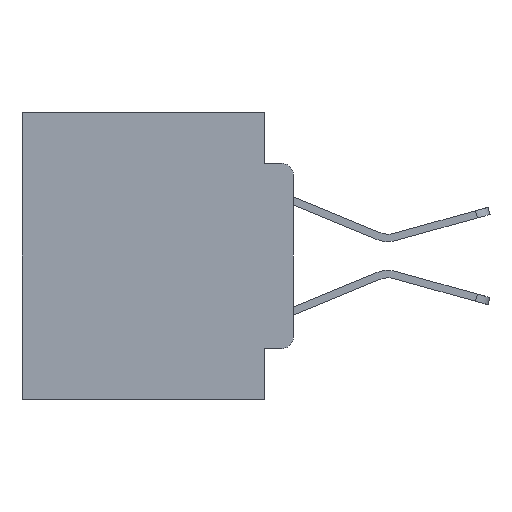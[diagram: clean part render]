
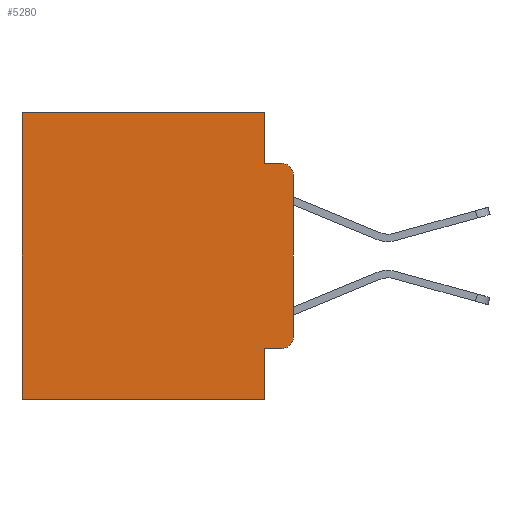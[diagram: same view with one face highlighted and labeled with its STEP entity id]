
A CAD part, left-side view. The second image highlights one B-rep face of the part: STEP entity #5280.
In plain terms, the highlighted planar face has unit normal (-1, 0, 0).
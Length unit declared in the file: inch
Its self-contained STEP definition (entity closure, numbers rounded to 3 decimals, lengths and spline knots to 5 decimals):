
#227 = LINE ( 'NONE', #12690, #11710 ) ;
#474 = LINE ( 'NONE', #9135, #16543 ) ;
#956 = VECTOR ( 'NONE', #20732, 39.37008 ) ;
#1120 = FACE_OUTER_BOUND ( 'NONE', #25612, .T. ) ;
#1221 = VECTOR ( 'NONE', #12861, 39.37008 ) ;
#1805 = VERTEX_POINT ( 'NONE', #17843 ) ;
#2134 = LINE ( 'NONE', #21038, #1221 ) ;
#2666 = LINE ( 'NONE', #25555, #8576 ) ;
#3154 = AXIS2_PLACEMENT_3D ( 'NONE', #25519, #4149, #27176 ) ;
#3446 = VERTEX_POINT ( 'NONE', #4887 ) ;
#3476 = EDGE_CURVE ( 'NONE', #4580, #18913, #23911, .T. ) ;
#3707 = LINE ( 'NONE', #9646, #15598 ) ;
#4149 = DIRECTION ( 'NONE',  ( -1., 0., 0. ) ) ;
#4408 = VERTEX_POINT ( 'NONE', #26683 ) ;
#4580 = VERTEX_POINT ( 'NONE', #16637 ) ;
#4743 = DIRECTION ( 'NONE',  ( 0., 0., -1. ) ) ;
#4791 = CARTESIAN_POINT ( 'NONE',  ( 0.298, 0.02, -0.1085 ) ) ;
#4887 = CARTESIAN_POINT ( 'NONE',  ( 0.298, 0.473, 0. ) ) ;
#5112 = VERTEX_POINT ( 'NONE', #25258 ) ;
#5280 = ADVANCED_FACE ( 'NONE', ( #1120 ), #5679, .F. ) ;
#5679 = PLANE ( 'NONE',  #7885 ) ;
#5736 = ORIENTED_EDGE ( 'NONE', *, *, #14434, .T. ) ;
#6062 = CARTESIAN_POINT ( 'NONE',  ( 0.298, 0.02, -0.0885 ) ) ;
#6555 = ORIENTED_EDGE ( 'NONE', *, *, #7432, .T. ) ;
#6926 = EDGE_CURVE ( 'NONE', #19111, #4408, #9971, .T. ) ;
#6990 = DIRECTION ( 'NONE',  ( 0., 0., -1. ) ) ;
#7391 = CARTESIAN_POINT ( 'NONE',  ( 0.298, 0.051, -0.4115 ) ) ;
#7432 = EDGE_CURVE ( 'NONE', #5112, #18913, #12860, .T. ) ;
#7465 = DIRECTION ( 'NONE',  ( 1., 0., 0. ) ) ;
#7572 = DIRECTION ( 'NONE',  ( 0., 1., 0. ) ) ;
#7725 = CARTESIAN_POINT ( 'NONE',  ( 0.298, 0., 0. ) ) ;
#7873 = LINE ( 'NONE', #12290, #956 ) ;
#7885 = AXIS2_PLACEMENT_3D ( 'NONE', #7725, #7465, #24417 ) ;
#8168 = CIRCLE ( 'NONE', #15637, 0.02 ) ;
#8372 = DIRECTION ( 'NONE',  ( 0., 0., -1. ) ) ;
#8576 = VECTOR ( 'NONE', #10661, 39.37008 ) ;
#8638 = EDGE_CURVE ( 'NONE', #24004, #5112, #7873, .T. ) ;
#8888 = CARTESIAN_POINT ( 'NONE',  ( 0.298, 0., 0. ) ) ;
#9005 = CARTESIAN_POINT ( 'NONE',  ( 0.298, 0., -0.3915 ) ) ;
#9135 = CARTESIAN_POINT ( 'NONE',  ( 0.298, 0.051, 0. ) ) ;
#9478 = ORIENTED_EDGE ( 'NONE', *, *, #25995, .F. ) ;
#9646 = CARTESIAN_POINT ( 'NONE',  ( 0.298, 0., 0. ) ) ;
#9971 = LINE ( 'NONE', #24458, #17268 ) ;
#10642 = CARTESIAN_POINT ( 'NONE',  ( 0.298, 0.473, -0.5 ) ) ;
#10661 = DIRECTION ( 'NONE',  ( 0., 1., 0. ) ) ;
#10952 = ORIENTED_EDGE ( 'NONE', *, *, #14062, .F. ) ;
#11213 = DIRECTION ( 'NONE',  ( 0., 0., -1. ) ) ;
#11501 = EDGE_CURVE ( 'NONE', #1805, #16860, #2666, .T. ) ;
#11696 = ORIENTED_EDGE ( 'NONE', *, *, #6926, .F. ) ;
#11710 = VECTOR ( 'NONE', #8372, 39.37008 ) ;
#11771 = VERTEX_POINT ( 'NONE', #6062 ) ;
#12290 = CARTESIAN_POINT ( 'NONE',  ( 0.298, 0.051, -0.4115 ) ) ;
#12690 = CARTESIAN_POINT ( 'NONE',  ( 0.298, 0.473, 0. ) ) ;
#12860 = CIRCLE ( 'NONE', #3154, 0.02 ) ;
#12861 = DIRECTION ( 'NONE',  ( 0., -1., 0. ) ) ;
#14062 = EDGE_CURVE ( 'NONE', #24004, #1805, #474, .T. ) ;
#14434 = EDGE_CURVE ( 'NONE', #3446, #16860, #227, .T. ) ;
#14589 = ORIENTED_EDGE ( 'NONE', *, *, #8638, .T. ) ;
#15179 = EDGE_CURVE ( 'NONE', #19111, #3446, #3707, .T. ) ;
#15598 = VECTOR ( 'NONE', #7572, 39.37008 ) ;
#15637 = AXIS2_PLACEMENT_3D ( 'NONE', #4791, #17326, #6990 ) ;
#16543 = VECTOR ( 'NONE', #4743, 39.37008 ) ;
#16637 = CARTESIAN_POINT ( 'NONE',  ( 0.298, 0., -0.1085 ) ) ;
#16860 = VERTEX_POINT ( 'NONE', #10642 ) ;
#17250 = EDGE_CURVE ( 'NONE', #4580, #11771, #8168, .T. ) ;
#17268 = VECTOR ( 'NONE', #26643, 39.37008 ) ;
#17326 = DIRECTION ( 'NONE',  ( -1., 0., 0. ) ) ;
#17843 = CARTESIAN_POINT ( 'NONE',  ( 0.298, 0.051, -0.5 ) ) ;
#18090 = ORIENTED_EDGE ( 'NONE', *, *, #17250, .T. ) ;
#18132 = ORIENTED_EDGE ( 'NONE', *, *, #3476, .F. ) ;
#18913 = VERTEX_POINT ( 'NONE', #9005 ) ;
#19111 = VERTEX_POINT ( 'NONE', #22512 ) ;
#20628 = ORIENTED_EDGE ( 'NONE', *, *, #11501, .F. ) ;
#20732 = DIRECTION ( 'NONE',  ( 0., -1., 0. ) ) ;
#20934 = ORIENTED_EDGE ( 'NONE', *, *, #15179, .T. ) ;
#21038 = CARTESIAN_POINT ( 'NONE',  ( 0.298, 0.051, -0.0885 ) ) ;
#22512 = CARTESIAN_POINT ( 'NONE',  ( 0.298, 0.051, 0. ) ) ;
#23911 = LINE ( 'NONE', #8888, #25512 ) ;
#24004 = VERTEX_POINT ( 'NONE', #7391 ) ;
#24417 = DIRECTION ( 'NONE',  ( 0., 0., -1. ) ) ;
#24458 = CARTESIAN_POINT ( 'NONE',  ( 0.298, 0.051, 0. ) ) ;
#25258 = CARTESIAN_POINT ( 'NONE',  ( 0.298, 0.02, -0.4115 ) ) ;
#25512 = VECTOR ( 'NONE', #11213, 39.37008 ) ;
#25519 = CARTESIAN_POINT ( 'NONE',  ( 0.298, 0.02, -0.3915 ) ) ;
#25555 = CARTESIAN_POINT ( 'NONE',  ( 0.298, 0., -0.5 ) ) ;
#25612 = EDGE_LOOP ( 'NONE', ( #18132, #18090, #9478, #11696, #20934, #5736, #20628, #10952, #14589, #6555 ) ) ;
#25995 = EDGE_CURVE ( 'NONE', #4408, #11771, #2134, .T. ) ;
#26643 = DIRECTION ( 'NONE',  ( 0., 0., -1. ) ) ;
#26683 = CARTESIAN_POINT ( 'NONE',  ( 0.298, 0.051, -0.0885 ) ) ;
#27176 = DIRECTION ( 'NONE',  ( 0., 0., -1. ) ) ;
